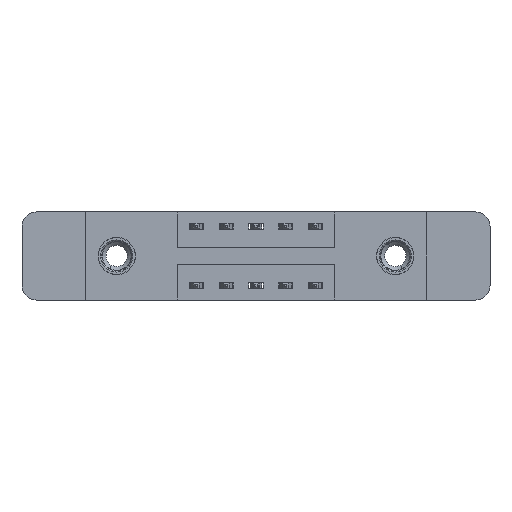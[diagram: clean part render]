
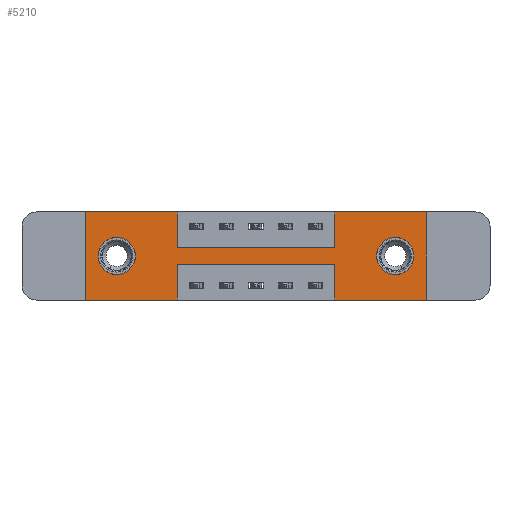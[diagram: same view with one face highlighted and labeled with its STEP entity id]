
A CAD part, front view. The second image highlights one B-rep face of the part: STEP entity #5210.
In plain terms, the highlighted planar face has unit normal (0, -1, 0).
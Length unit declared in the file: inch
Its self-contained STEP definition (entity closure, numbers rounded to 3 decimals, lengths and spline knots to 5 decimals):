
#151 = DIRECTION ( 'NONE',  ( -1., 0., 0. ) ) ;
#247 = VECTOR ( 'NONE', #972, 39.37008 ) ;
#352 = EDGE_CURVE ( 'NONE', #12498, #9823, #13347, .T. ) ;
#653 = VECTOR ( 'NONE', #8445, 39.37008 ) ;
#789 = VERTEX_POINT ( 'NONE', #13122 ) ;
#813 = CARTESIAN_POINT ( 'NONE',  ( 1.435, 0., -0.37 ) ) ;
#830 = DIRECTION ( 'NONE',  ( -1., 0., 0. ) ) ;
#843 = CARTESIAN_POINT ( 'NONE',  ( 1.0475, 0., -0.22 ) ) ;
#893 = CARTESIAN_POINT ( 'NONE',  ( 0.3875, 0., -0.37 ) ) ;
#909 = VECTOR ( 'NONE', #12821, 39.37008 ) ;
#934 = CARTESIAN_POINT ( 'NONE',  ( 1.0475, 0., 0. ) ) ;
#972 = DIRECTION ( 'NONE',  ( 0., 0., 1. ) ) ;
#979 = CARTESIAN_POINT ( 'NONE',  ( 0., 0., -0.37 ) ) ;
#1188 = DIRECTION ( 'NONE',  ( 0., 1., 0. ) ) ;
#1603 = DIRECTION ( 'NONE',  ( 1., 0., 0. ) ) ;
#1608 = ORIENTED_EDGE ( 'NONE', *, *, #10836, .T. ) ;
#1615 = EDGE_CURVE ( 'NONE', #6739, #12345, #7276, .T. ) ;
#1646 = DIRECTION ( 'NONE',  ( 0., 0., 1. ) ) ;
#1820 = CARTESIAN_POINT ( 'NONE',  ( 1.3025, 0., -0.107 ) ) ;
#1937 = VERTEX_POINT ( 'NONE', #12561 ) ;
#1971 = LINE ( 'NONE', #4690, #2811 ) ;
#2084 = DIRECTION ( 'NONE',  ( 0., -1., 0. ) ) ;
#2149 = CIRCLE ( 'NONE', #6662, 0.078 ) ;
#2190 = CARTESIAN_POINT ( 'NONE',  ( 0.1325, 0., -0.263 ) ) ;
#2366 = VECTOR ( 'NONE', #151, 39.37008 ) ;
#2537 = CARTESIAN_POINT ( 'NONE',  ( 1.3025, 0., -0.185 ) ) ;
#2616 = CARTESIAN_POINT ( 'NONE',  ( 1.435, 0., 0. ) ) ;
#2811 = VECTOR ( 'NONE', #1603, 39.37008 ) ;
#2883 = FACE_OUTER_BOUND ( 'NONE', #10539, .T. ) ;
#2981 = EDGE_CURVE ( 'NONE', #9823, #789, #4083, .T. ) ;
#3113 = DIRECTION ( 'NONE',  ( 0., 0., -1. ) ) ;
#3144 = CARTESIAN_POINT ( 'NONE',  ( 0., 0., -0.37 ) ) ;
#3203 = EDGE_CURVE ( 'NONE', #4547, #8070, #13107, .T. ) ;
#3401 = ORIENTED_EDGE ( 'NONE', *, *, #3203, .F. ) ;
#3524 = FACE_BOUND ( 'NONE', #6745, .T. ) ;
#4035 = ORIENTED_EDGE ( 'NONE', *, *, #11858, .T. ) ;
#4083 = LINE ( 'NONE', #3144, #653 ) ;
#4178 = EDGE_CURVE ( 'NONE', #9053, #11991, #12711, .T. ) ;
#4291 = AXIS2_PLACEMENT_3D ( 'NONE', #10822, #4663, #4566 ) ;
#4471 = ORIENTED_EDGE ( 'NONE', *, *, #10118, .F. ) ;
#4547 = VERTEX_POINT ( 'NONE', #10384 ) ;
#4566 = DIRECTION ( 'NONE',  ( 0., 0., -1. ) ) ;
#4634 = CARTESIAN_POINT ( 'NONE',  ( 0.3875, 0., 0. ) ) ;
#4649 = FACE_BOUND ( 'NONE', #11184, .T. ) ;
#4663 = DIRECTION ( 'NONE',  ( 0., 1., 0. ) ) ;
#4690 = CARTESIAN_POINT ( 'NONE',  ( 0., 0., 0. ) ) ;
#4870 = VERTEX_POINT ( 'NONE', #2190 ) ;
#5065 = LINE ( 'NONE', #4634, #9283 ) ;
#5088 = VECTOR ( 'NONE', #7734, 39.37008 ) ;
#5157 = LINE ( 'NONE', #8451, #11845 ) ;
#5210 = ADVANCED_FACE ( 'NONE', ( #3524, #4649, #2883 ), #6171, .T. ) ;
#5496 = EDGE_CURVE ( 'NONE', #6105, #4870, #2149, .T. ) ;
#5553 = ORIENTED_EDGE ( 'NONE', *, *, #1615, .F. ) ;
#5622 = CARTESIAN_POINT ( 'NONE',  ( 0.3875, 0., -0.37 ) ) ;
#5762 = CARTESIAN_POINT ( 'NONE',  ( 0., 0., -0.37 ) ) ;
#5778 = DIRECTION ( 'NONE',  ( 0., 0., 1. ) ) ;
#6105 = VERTEX_POINT ( 'NONE', #9267 ) ;
#6138 = AXIS2_PLACEMENT_3D ( 'NONE', #979, #2084, #3113 ) ;
#6171 = PLANE ( 'NONE',  #6138 ) ;
#6177 = CARTESIAN_POINT ( 'NONE',  ( 1.3025, 0., -0.263 ) ) ;
#6344 = ORIENTED_EDGE ( 'NONE', *, *, #2981, .F. ) ;
#6662 = AXIS2_PLACEMENT_3D ( 'NONE', #7322, #1188, #5778 ) ;
#6695 = DIRECTION ( 'NONE',  ( 0., 1., 0. ) ) ;
#6739 = VERTEX_POINT ( 'NONE', #893 ) ;
#6745 = EDGE_LOOP ( 'NONE', ( #1608, #4035 ) ) ;
#7276 = LINE ( 'NONE', #5762, #8924 ) ;
#7305 = CARTESIAN_POINT ( 'NONE',  ( 0., 0., 0. ) ) ;
#7322 = CARTESIAN_POINT ( 'NONE',  ( 0.1325, 0., -0.185 ) ) ;
#7401 = LINE ( 'NONE', #5622, #909 ) ;
#7408 = EDGE_CURVE ( 'NONE', #1937, #6739, #7401, .T. ) ;
#7620 = CARTESIAN_POINT ( 'NONE',  ( 0., 0., -0.37 ) ) ;
#7734 = DIRECTION ( 'NONE',  ( 1., 0., 0. ) ) ;
#7842 = VECTOR ( 'NONE', #9900, 39.37008 ) ;
#7886 = VERTEX_POINT ( 'NONE', #12379 ) ;
#7901 = LINE ( 'NONE', #10438, #2366 ) ;
#7960 = ORIENTED_EDGE ( 'NONE', *, *, #9614, .T. ) ;
#7990 = CIRCLE ( 'NONE', #4291, 0.078 ) ;
#8070 = VERTEX_POINT ( 'NONE', #12050 ) ;
#8102 = VECTOR ( 'NONE', #1646, 39.37008 ) ;
#8228 = EDGE_CURVE ( 'NONE', #8665, #1937, #7901, .T. ) ;
#8445 = DIRECTION ( 'NONE',  ( -1., 0., 0. ) ) ;
#8451 = CARTESIAN_POINT ( 'NONE',  ( 1.0475, 0., -0.37 ) ) ;
#8524 = CARTESIAN_POINT ( 'NONE',  ( 0.1325, 0., -0.185 ) ) ;
#8528 = EDGE_CURVE ( 'NONE', #7886, #4547, #13227, .T. ) ;
#8665 = VERTEX_POINT ( 'NONE', #843 ) ;
#8854 = LINE ( 'NONE', #13394, #247 ) ;
#8924 = VECTOR ( 'NONE', #830, 39.37008 ) ;
#8947 = ORIENTED_EDGE ( 'NONE', *, *, #10244, .F. ) ;
#9005 = ORIENTED_EDGE ( 'NONE', *, *, #5496, .T. ) ;
#9050 = VERTEX_POINT ( 'NONE', #1820 ) ;
#9053 = VERTEX_POINT ( 'NONE', #13279 ) ;
#9267 = CARTESIAN_POINT ( 'NONE',  ( 0.1325, 0., -0.107 ) ) ;
#9283 = VECTOR ( 'NONE', #10024, 39.37008 ) ;
#9428 = CIRCLE ( 'NONE', #12954, 0.078 ) ;
#9456 = EDGE_CURVE ( 'NONE', #11991, #7886, #5065, .T. ) ;
#9575 = DIRECTION ( 'NONE',  ( 0., 1., 0. ) ) ;
#9614 = EDGE_CURVE ( 'NONE', #4870, #6105, #13377, .T. ) ;
#9817 = DIRECTION ( 'NONE',  ( 0., 0., -1. ) ) ;
#9823 = VERTEX_POINT ( 'NONE', #813 ) ;
#9900 = DIRECTION ( 'NONE',  ( 0., 0., -1. ) ) ;
#10024 = DIRECTION ( 'NONE',  ( 0., 0., -1. ) ) ;
#10118 = EDGE_CURVE ( 'NONE', #12345, #9053, #8854, .T. ) ;
#10146 = DIRECTION ( 'NONE',  ( 1., 0., 0. ) ) ;
#10166 = ORIENTED_EDGE ( 'NONE', *, *, #4178, .F. ) ;
#10244 = EDGE_CURVE ( 'NONE', #789, #8665, #5157, .T. ) ;
#10274 = ORIENTED_EDGE ( 'NONE', *, *, #9456, .F. ) ;
#10284 = ORIENTED_EDGE ( 'NONE', *, *, #7408, .F. ) ;
#10302 = AXIS2_PLACEMENT_3D ( 'NONE', #8524, #9575, #12547 ) ;
#10384 = CARTESIAN_POINT ( 'NONE',  ( 1.0475, 0., -0.15 ) ) ;
#10385 = VERTEX_POINT ( 'NONE', #6177 ) ;
#10438 = CARTESIAN_POINT ( 'NONE',  ( 0.3875, 0., -0.22 ) ) ;
#10475 = ORIENTED_EDGE ( 'NONE', *, *, #8228, .F. ) ;
#10502 = VECTOR ( 'NONE', #10146, 39.37008 ) ;
#10539 = EDGE_LOOP ( 'NONE', ( #10284, #10475, #8947, #6344, #11528, #10540, #3401, #10858, #10274, #10166, #4471, #5553 ) ) ;
#10540 = ORIENTED_EDGE ( 'NONE', *, *, #12444, .F. ) ;
#10822 = CARTESIAN_POINT ( 'NONE',  ( 1.3025, 0., -0.185 ) ) ;
#10836 = EDGE_CURVE ( 'NONE', #9050, #10385, #9428, .T. ) ;
#10858 = ORIENTED_EDGE ( 'NONE', *, *, #8528, .F. ) ;
#11184 = EDGE_LOOP ( 'NONE', ( #9005, #7960 ) ) ;
#11528 = ORIENTED_EDGE ( 'NONE', *, *, #352, .F. ) ;
#11681 = DIRECTION ( 'NONE',  ( 0., 0., 1. ) ) ;
#11845 = VECTOR ( 'NONE', #11681, 39.37008 ) ;
#11858 = EDGE_CURVE ( 'NONE', #10385, #9050, #7990, .T. ) ;
#11991 = VERTEX_POINT ( 'NONE', #12145 ) ;
#12050 = CARTESIAN_POINT ( 'NONE',  ( 1.0475, 0., 0. ) ) ;
#12145 = CARTESIAN_POINT ( 'NONE',  ( 0.3875, 0., 0. ) ) ;
#12345 = VERTEX_POINT ( 'NONE', #7620 ) ;
#12379 = CARTESIAN_POINT ( 'NONE',  ( 0.3875, 0., -0.15 ) ) ;
#12444 = EDGE_CURVE ( 'NONE', #8070, #12498, #1971, .T. ) ;
#12498 = VERTEX_POINT ( 'NONE', #13134 ) ;
#12547 = DIRECTION ( 'NONE',  ( 0., 0., 1. ) ) ;
#12561 = CARTESIAN_POINT ( 'NONE',  ( 0.3875, 0., -0.22 ) ) ;
#12711 = LINE ( 'NONE', #7305, #5088 ) ;
#12821 = DIRECTION ( 'NONE',  ( 0., 0., -1. ) ) ;
#12954 = AXIS2_PLACEMENT_3D ( 'NONE', #2537, #6695, #9817 ) ;
#13107 = LINE ( 'NONE', #934, #8102 ) ;
#13113 = CARTESIAN_POINT ( 'NONE',  ( 0.3875, 0., -0.15 ) ) ;
#13122 = CARTESIAN_POINT ( 'NONE',  ( 1.0475, 0., -0.37 ) ) ;
#13134 = CARTESIAN_POINT ( 'NONE',  ( 1.435, 0., 0. ) ) ;
#13227 = LINE ( 'NONE', #13113, #10502 ) ;
#13279 = CARTESIAN_POINT ( 'NONE',  ( 0., 0., 0. ) ) ;
#13347 = LINE ( 'NONE', #2616, #7842 ) ;
#13377 = CIRCLE ( 'NONE', #10302, 0.078 ) ;
#13394 = CARTESIAN_POINT ( 'NONE',  ( 0., 0., 0. ) ) ;
